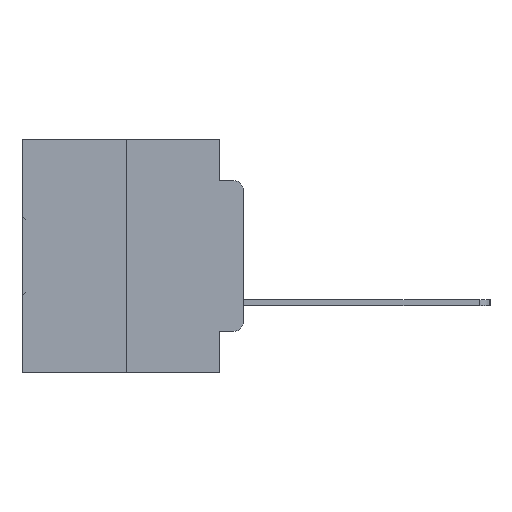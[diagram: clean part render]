
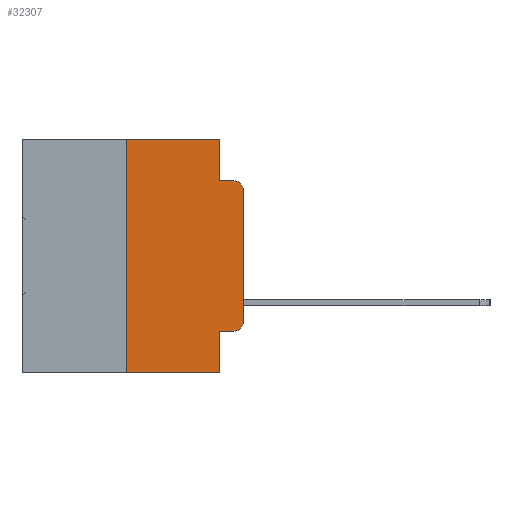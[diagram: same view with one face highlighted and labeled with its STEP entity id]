
A CAD part, left-side view. The second image highlights one B-rep face of the part: STEP entity #32307.
In plain terms, the highlighted planar face has unit normal (-1, 0, 0).
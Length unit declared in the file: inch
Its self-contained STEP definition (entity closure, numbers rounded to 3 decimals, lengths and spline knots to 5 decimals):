
#1304 = CARTESIAN_POINT ( 'NONE',  ( 0., 0.473, -0.5 ) ) ;
#1633 = ORIENTED_EDGE ( 'NONE', *, *, #6962, .F. ) ;
#2046 = DIRECTION ( 'NONE',  ( 0., -1., 0. ) ) ;
#2162 = CARTESIAN_POINT ( 'NONE',  ( 0., 0., -0.1085 ) ) ;
#2349 = EDGE_CURVE ( 'NONE', #3572, #24956, #17309, .T. ) ;
#2689 = VECTOR ( 'NONE', #28290, 39.37008 ) ;
#3117 = CARTESIAN_POINT ( 'NONE',  ( 0., 0.02, -0.4115 ) ) ;
#3516 = CARTESIAN_POINT ( 'NONE',  ( 0., 0., -0.3915 ) ) ;
#3572 = VERTEX_POINT ( 'NONE', #3516 ) ;
#3859 = VECTOR ( 'NONE', #13569, 39.37008 ) ;
#3970 = CARTESIAN_POINT ( 'NONE',  ( 0., 0.02, -0.1085 ) ) ;
#4057 = DIRECTION ( 'NONE',  ( 0., -1., 0. ) ) ;
#4108 = CARTESIAN_POINT ( 'NONE',  ( 0., 0.051, -0.0885 ) ) ;
#4165 = CIRCLE ( 'NONE', #34114, 0.02 ) ;
#4780 = DIRECTION ( 'NONE',  ( 0., 0., 1. ) ) ;
#6678 = DIRECTION ( 'NONE',  ( 0., 0., -1. ) ) ;
#6962 = EDGE_CURVE ( 'NONE', #21073, #28734, #10980, .T. ) ;
#7108 = AXIS2_PLACEMENT_3D ( 'NONE', #3970, #22975, #6678 ) ;
#7568 = VECTOR ( 'NONE', #10759, 39.37008 ) ;
#7593 = ORIENTED_EDGE ( 'NONE', *, *, #34631, .T. ) ;
#7604 = DIRECTION ( 'NONE',  ( -1., 0., 0. ) ) ;
#8051 = ORIENTED_EDGE ( 'NONE', *, *, #2349, .T. ) ;
#8389 = VECTOR ( 'NONE', #2046, 39.37008 ) ;
#8829 = FACE_OUTER_BOUND ( 'NONE', #32951, .T. ) ;
#9115 = LINE ( 'NONE', #32374, #15478 ) ;
#9403 = VECTOR ( 'NONE', #4057, 39.37008 ) ;
#10067 = VECTOR ( 'NONE', #4780, 39.37008 ) ;
#10240 = LINE ( 'NONE', #1304, #9403 ) ;
#10759 = DIRECTION ( 'NONE',  ( 0., 0., -1. ) ) ;
#10980 = LINE ( 'NONE', #18904, #3859 ) ;
#12034 = CARTESIAN_POINT ( 'NONE',  ( 0., 0.473, 0. ) ) ;
#12451 = VECTOR ( 'NONE', #17641, 39.37008 ) ;
#13137 = ORIENTED_EDGE ( 'NONE', *, *, #30357, .T. ) ;
#13569 = DIRECTION ( 'NONE',  ( 0., 0., 1. ) ) ;
#13924 = EDGE_CURVE ( 'NONE', #14951, #17987, #9115, .T. ) ;
#14463 = EDGE_CURVE ( 'NONE', #16751, #3572, #4165, .T. ) ;
#14505 = CARTESIAN_POINT ( 'NONE',  ( 0., 0.25, -0.5 ) ) ;
#14757 = LINE ( 'NONE', #21757, #7568 ) ;
#14951 = VERTEX_POINT ( 'NONE', #23193 ) ;
#14989 = ORIENTED_EDGE ( 'NONE', *, *, #28623, .T. ) ;
#15395 = CARTESIAN_POINT ( 'NONE',  ( 0., 0.051, -0.0885 ) ) ;
#15478 = VECTOR ( 'NONE', #16274, 39.37008 ) ;
#16274 = DIRECTION ( 'NONE',  ( 0., 0., -1. ) ) ;
#16285 = ORIENTED_EDGE ( 'NONE', *, *, #13924, .F. ) ;
#16448 = LINE ( 'NONE', #15395, #8389 ) ;
#16751 = VERTEX_POINT ( 'NONE', #3117 ) ;
#17309 = LINE ( 'NONE', #20990, #10067 ) ;
#17641 = DIRECTION ( 'NONE',  ( 0., -1., 0. ) ) ;
#17987 = VERTEX_POINT ( 'NONE', #21902 ) ;
#18531 = ORIENTED_EDGE ( 'NONE', *, *, #20169, .F. ) ;
#18679 = DIRECTION ( 'NONE',  ( 0., 0., -1. ) ) ;
#18828 = ORIENTED_EDGE ( 'NONE', *, *, #20115, .F. ) ;
#18904 = CARTESIAN_POINT ( 'NONE',  ( 0., 0.25, 0. ) ) ;
#19256 = VERTEX_POINT ( 'NONE', #27933 ) ;
#20115 = EDGE_CURVE ( 'NONE', #21725, #19256, #16448, .T. ) ;
#20169 = EDGE_CURVE ( 'NONE', #32767, #21725, #14757, .T. ) ;
#20411 = ORIENTED_EDGE ( 'NONE', *, *, #23638, .F. ) ;
#20990 = CARTESIAN_POINT ( 'NONE',  ( 0., 0., 0. ) ) ;
#21073 = VERTEX_POINT ( 'NONE', #14505 ) ;
#21725 = VERTEX_POINT ( 'NONE', #4108 ) ;
#21757 = CARTESIAN_POINT ( 'NONE',  ( 0., 0.051, 0. ) ) ;
#21902 = CARTESIAN_POINT ( 'NONE',  ( 0., 0.051, -0.5 ) ) ;
#22975 = DIRECTION ( 'NONE',  ( -1., 0., 0. ) ) ;
#23193 = CARTESIAN_POINT ( 'NONE',  ( 0., 0.051, -0.4115 ) ) ;
#23484 = AXIS2_PLACEMENT_3D ( 'NONE', #29404, #34710, #18679 ) ;
#23638 = EDGE_CURVE ( 'NONE', #28734, #32767, #24362, .T. ) ;
#23914 = CARTESIAN_POINT ( 'NONE',  ( 0., 0.02, -0.3915 ) ) ;
#24362 = LINE ( 'NONE', #12034, #2689 ) ;
#24956 = VERTEX_POINT ( 'NONE', #2162 ) ;
#26086 = LINE ( 'NONE', #33707, #12451 ) ;
#26593 = DIRECTION ( 'NONE',  ( 0., 0., -1. ) ) ;
#26801 = CIRCLE ( 'NONE', #7108, 0.02 ) ;
#27933 = CARTESIAN_POINT ( 'NONE',  ( 0., 0.02, -0.0885 ) ) ;
#28290 = DIRECTION ( 'NONE',  ( 0., -1., 0. ) ) ;
#28623 = EDGE_CURVE ( 'NONE', #14951, #16751, #26086, .T. ) ;
#28734 = VERTEX_POINT ( 'NONE', #31380 ) ;
#29404 = CARTESIAN_POINT ( 'NONE',  ( 0., 0.473, 0. ) ) ;
#30357 = EDGE_CURVE ( 'NONE', #21073, #17987, #10240, .T. ) ;
#31380 = CARTESIAN_POINT ( 'NONE',  ( 0., 0.25, 0. ) ) ;
#32026 = PLANE ( 'NONE',  #23484 ) ;
#32307 = ADVANCED_FACE ( 'NONE', ( #8829 ), #32026, .F. ) ;
#32374 = CARTESIAN_POINT ( 'NONE',  ( 0., 0.051, 0. ) ) ;
#32767 = VERTEX_POINT ( 'NONE', #34209 ) ;
#32951 = EDGE_LOOP ( 'NONE', ( #8051, #7593, #18828, #18531, #20411, #1633, #13137, #16285, #14989, #34865 ) ) ;
#33707 = CARTESIAN_POINT ( 'NONE',  ( 0., 0.051, -0.4115 ) ) ;
#34114 = AXIS2_PLACEMENT_3D ( 'NONE', #23914, #7604, #26593 ) ;
#34209 = CARTESIAN_POINT ( 'NONE',  ( 0., 0.051, 0. ) ) ;
#34631 = EDGE_CURVE ( 'NONE', #24956, #19256, #26801, .T. ) ;
#34710 = DIRECTION ( 'NONE',  ( 1., 0., 0. ) ) ;
#34865 = ORIENTED_EDGE ( 'NONE', *, *, #14463, .T. ) ;
